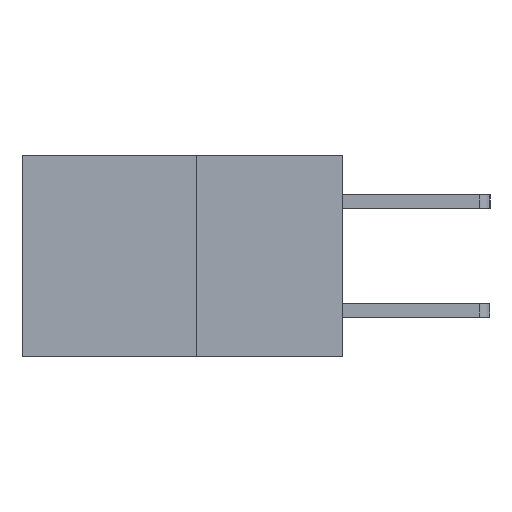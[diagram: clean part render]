
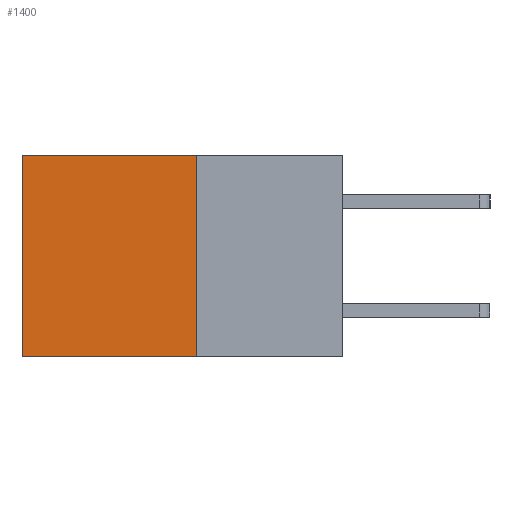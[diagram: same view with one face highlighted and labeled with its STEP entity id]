
A CAD part, left-side view. The second image highlights one B-rep face of the part: STEP entity #1400.
In plain terms, the highlighted planar face has unit normal (-1, 0, 0).
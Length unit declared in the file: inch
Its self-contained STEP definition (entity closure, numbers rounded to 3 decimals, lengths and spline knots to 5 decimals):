
#602 = EDGE_CURVE ( 'NONE', #4004, #1532, #7605, .T. ) ;
#1087 = EDGE_CURVE ( 'NONE', #2452, #4004, #2295, .T. ) ;
#1400 = ADVANCED_FACE ( 'NONE', ( #4840 ), #5595, .F. ) ;
#1532 = VERTEX_POINT ( 'NONE', #8684 ) ;
#1983 = ORIENTED_EDGE ( 'NONE', *, *, #3390, .F. ) ;
#2167 = VECTOR ( 'NONE', #8493, 39.37008 ) ;
#2278 = ORIENTED_EDGE ( 'NONE', *, *, #1087, .T. ) ;
#2295 = LINE ( 'NONE', #2687, #4398 ) ;
#2452 = VERTEX_POINT ( 'NONE', #2865 ) ;
#2687 = CARTESIAN_POINT ( 'NONE',  ( 0.277, 0.27, 0. ) ) ;
#2865 = CARTESIAN_POINT ( 'NONE',  ( 0.277, 0.27, 0. ) ) ;
#3044 = DIRECTION ( 'NONE',  ( 0., 1., 0. ) ) ;
#3313 = CARTESIAN_POINT ( 'NONE',  ( 0.277, 0.59, -0.37 ) ) ;
#3390 = EDGE_CURVE ( 'NONE', #8080, #1532, #8270, .T. ) ;
#4004 = VERTEX_POINT ( 'NONE', #8120 ) ;
#4398 = VECTOR ( 'NONE', #3044, 39.37008 ) ;
#4772 = CARTESIAN_POINT ( 'NONE',  ( 0.277, 0.27, -0.37 ) ) ;
#4840 = FACE_OUTER_BOUND ( 'NONE', #4957, .T. ) ;
#4856 = CARTESIAN_POINT ( 'NONE',  ( 0.277, 0.27, -0.37 ) ) ;
#4891 = DIRECTION ( 'NONE',  ( 0., 0., -1. ) ) ;
#4957 = EDGE_LOOP ( 'NONE', ( #7698, #1983, #6053, #2278 ) ) ;
#5143 = DIRECTION ( 'NONE',  ( 1., 0., 0. ) ) ;
#5595 = PLANE ( 'NONE',  #6139 ) ;
#5880 = EDGE_CURVE ( 'NONE', #2452, #8080, #7577, .T. ) ;
#6034 = DIRECTION ( 'NONE',  ( 0., 0., -1. ) ) ;
#6053 = ORIENTED_EDGE ( 'NONE', *, *, #5880, .F. ) ;
#6139 = AXIS2_PLACEMENT_3D ( 'NONE', #9642, #5143, #6034 ) ;
#6761 = CARTESIAN_POINT ( 'NONE',  ( 0.277, 0.27, -0.37 ) ) ;
#7302 = VECTOR ( 'NONE', #7487, 39.37008 ) ;
#7487 = DIRECTION ( 'NONE',  ( 0., 1., 0. ) ) ;
#7577 = LINE ( 'NONE', #4856, #8906 ) ;
#7605 = LINE ( 'NONE', #3313, #2167 ) ;
#7698 = ORIENTED_EDGE ( 'NONE', *, *, #602, .T. ) ;
#8080 = VERTEX_POINT ( 'NONE', #4772 ) ;
#8120 = CARTESIAN_POINT ( 'NONE',  ( 0.277, 0.59, 0. ) ) ;
#8270 = LINE ( 'NONE', #6761, #7302 ) ;
#8493 = DIRECTION ( 'NONE',  ( 0., 0., -1. ) ) ;
#8684 = CARTESIAN_POINT ( 'NONE',  ( 0.277, 0.59, -0.37 ) ) ;
#8906 = VECTOR ( 'NONE', #4891, 39.37008 ) ;
#9642 = CARTESIAN_POINT ( 'NONE',  ( 0.277, 0.27, -0.37 ) ) ;
